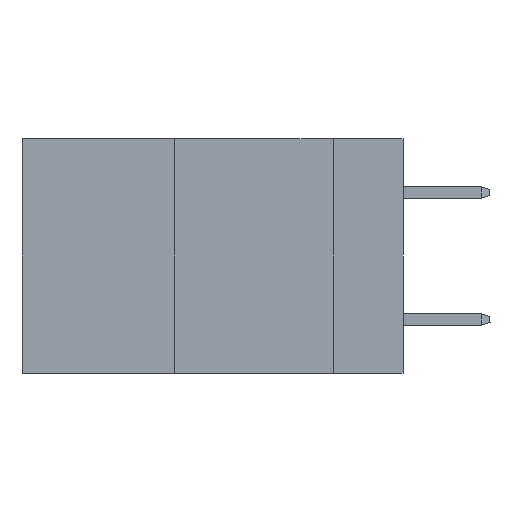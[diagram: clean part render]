
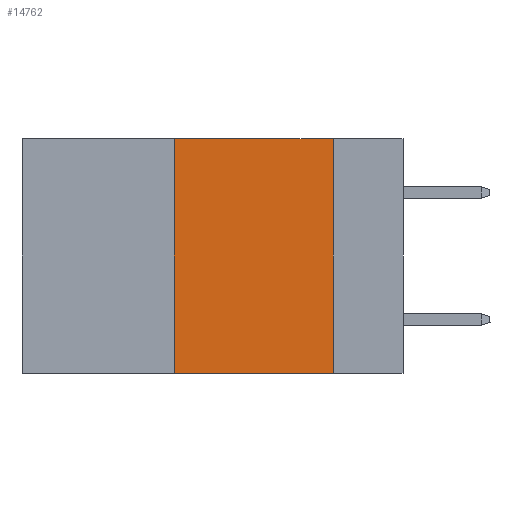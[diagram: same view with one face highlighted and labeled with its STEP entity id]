
A CAD part, left-side view. The second image highlights one B-rep face of the part: STEP entity #14762.
In plain terms, the highlighted planar face has unit normal (-1, 0, 0).
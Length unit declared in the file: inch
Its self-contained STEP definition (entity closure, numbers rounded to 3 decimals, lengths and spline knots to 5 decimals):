
#858 = EDGE_CURVE ( 'NONE', #30234, #4913, #6840, .T. ) ;
#1205 = DIRECTION ( 'NONE',  ( 0., 0., 1. ) ) ;
#1603 = VECTOR ( 'NONE', #2110, 39.37008 ) ;
#1885 = CARTESIAN_POINT ( 'NONE',  ( 0., 0.6, 0. ) ) ;
#2110 = DIRECTION ( 'NONE',  ( 0., 0., -1. ) ) ;
#2278 = ORIENTED_EDGE ( 'NONE', *, *, #13812, .F. ) ;
#4913 = VERTEX_POINT ( 'NONE', #15329 ) ;
#6840 = LINE ( 'NONE', #14078, #1603 ) ;
#8219 = DIRECTION ( 'NONE',  ( 0., -1., 0. ) ) ;
#8435 = FACE_OUTER_BOUND ( 'NONE', #10755, .T. ) ;
#9344 = EDGE_CURVE ( 'NONE', #29611, #4913, #11223, .T. ) ;
#9958 = EDGE_CURVE ( 'NONE', #21651, #30234, #26403, .T. ) ;
#10755 = EDGE_LOOP ( 'NONE', ( #23489, #23913, #2278, #27965 ) ) ;
#11223 = LINE ( 'NONE', #13559, #22497 ) ;
#12543 = DIRECTION ( 'NONE',  ( 1., 0., 0. ) ) ;
#13004 = PLANE ( 'NONE',  #14533 ) ;
#13559 = CARTESIAN_POINT ( 'NONE',  ( 0., 0.6, -0.37 ) ) ;
#13812 = EDGE_CURVE ( 'NONE', #29611, #21651, #22871, .T. ) ;
#14078 = CARTESIAN_POINT ( 'NONE',  ( 0., 0.11, 0. ) ) ;
#14533 = AXIS2_PLACEMENT_3D ( 'NONE', #29499, #12543, #18060 ) ;
#14762 = ADVANCED_FACE ( 'NONE', ( #8435 ), #13004, .F. ) ;
#15329 = CARTESIAN_POINT ( 'NONE',  ( 0., 0.11, -0.37 ) ) ;
#16787 = CARTESIAN_POINT ( 'NONE',  ( 0., 0.11, 0. ) ) ;
#18060 = DIRECTION ( 'NONE',  ( 0., 0., -1. ) ) ;
#19982 = VECTOR ( 'NONE', #21160, 39.37008 ) ;
#20215 = VECTOR ( 'NONE', #1205, 39.37008 ) ;
#21160 = DIRECTION ( 'NONE',  ( 0., -1., 0. ) ) ;
#21651 = VERTEX_POINT ( 'NONE', #22464 ) ;
#22464 = CARTESIAN_POINT ( 'NONE',  ( 0., 0.36, 0. ) ) ;
#22497 = VECTOR ( 'NONE', #8219, 39.37008 ) ;
#22871 = LINE ( 'NONE', #28199, #20215 ) ;
#23489 = ORIENTED_EDGE ( 'NONE', *, *, #858, .F. ) ;
#23696 = CARTESIAN_POINT ( 'NONE',  ( 0., 0.36, -0.37 ) ) ;
#23913 = ORIENTED_EDGE ( 'NONE', *, *, #9958, .F. ) ;
#26403 = LINE ( 'NONE', #1885, #19982 ) ;
#27965 = ORIENTED_EDGE ( 'NONE', *, *, #9344, .T. ) ;
#28199 = CARTESIAN_POINT ( 'NONE',  ( 0., 0.36, 0. ) ) ;
#29499 = CARTESIAN_POINT ( 'NONE',  ( 0., 0.6, 0. ) ) ;
#29611 = VERTEX_POINT ( 'NONE', #23696 ) ;
#30234 = VERTEX_POINT ( 'NONE', #16787 ) ;
